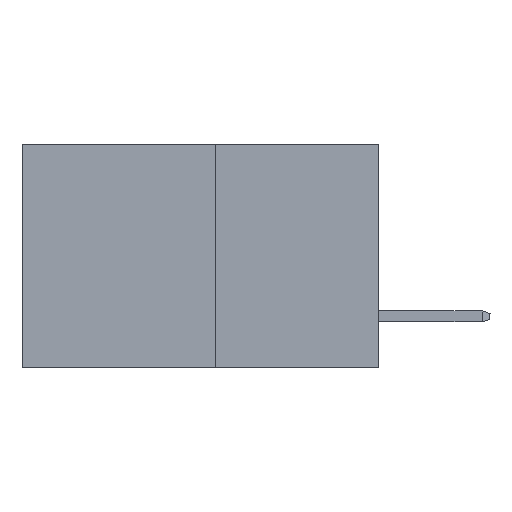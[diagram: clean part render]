
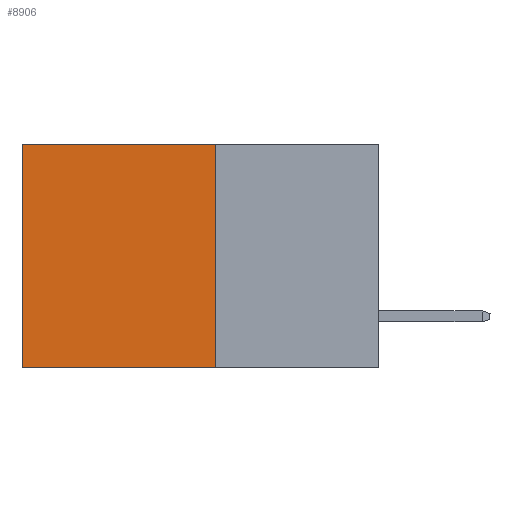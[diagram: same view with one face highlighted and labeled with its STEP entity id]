
A CAD part, left-side view. The second image highlights one B-rep face of the part: STEP entity #8906.
In plain terms, the highlighted planar face has unit normal (-1, 0, 0).
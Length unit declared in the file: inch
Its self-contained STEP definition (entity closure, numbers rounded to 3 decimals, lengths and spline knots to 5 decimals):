
#90 = ORIENTED_EDGE ( 'NONE', *, *, #6426, .F. ) ;
#382 = LINE ( 'NONE', #3004, #10397 ) ;
#418 = EDGE_CURVE ( 'NONE', #11303, #11766, #382, .T. ) ;
#494 = LINE ( 'NONE', #7568, #8043 ) ;
#1025 = LINE ( 'NONE', #3298, #10951 ) ;
#1126 = CARTESIAN_POINT ( 'NONE',  ( 0.277, 0.27, 0. ) ) ;
#1279 = EDGE_CURVE ( 'NONE', #1884, #5634, #1025, .T. ) ;
#1542 = ORIENTED_EDGE ( 'NONE', *, *, #1279, .T. ) ;
#1884 = VERTEX_POINT ( 'NONE', #11055 ) ;
#2034 = DIRECTION ( 'NONE',  ( 0., 1., 0. ) ) ;
#2112 = ORIENTED_EDGE ( 'NONE', *, *, #418, .F. ) ;
#2832 = CARTESIAN_POINT ( 'NONE',  ( 0.277, 0.59, -0.37 ) ) ;
#3004 = CARTESIAN_POINT ( 'NONE',  ( 0.277, 0.27, -0.37 ) ) ;
#3298 = CARTESIAN_POINT ( 'NONE',  ( 0.277, 0.59, -0.37 ) ) ;
#3558 = AXIS2_PLACEMENT_3D ( 'NONE', #8500, #8490, #8481 ) ;
#3573 = CARTESIAN_POINT ( 'NONE',  ( 0.277, 0.27, -0.37 ) ) ;
#4553 = FACE_OUTER_BOUND ( 'NONE', #7963, .T. ) ;
#4864 = EDGE_CURVE ( 'NONE', #11303, #1884, #494, .T. ) ;
#5371 = DIRECTION ( 'NONE',  ( 0., 0., -1. ) ) ;
#5634 = VERTEX_POINT ( 'NONE', #2832 ) ;
#5747 = DIRECTION ( 'NONE',  ( 0., 1., 0. ) ) ;
#6426 = EDGE_CURVE ( 'NONE', #11766, #5634, #8296, .T. ) ;
#7568 = CARTESIAN_POINT ( 'NONE',  ( 0.277, 0.27, 0. ) ) ;
#7963 = EDGE_LOOP ( 'NONE', ( #1542, #90, #2112, #10180 ) ) ;
#8020 = VECTOR ( 'NONE', #2034, 39.37008 ) ;
#8043 = VECTOR ( 'NONE', #5747, 39.37008 ) ;
#8296 = LINE ( 'NONE', #3573, #8020 ) ;
#8481 = DIRECTION ( 'NONE',  ( 0., 0., -1. ) ) ;
#8490 = DIRECTION ( 'NONE',  ( 1., 0., 0. ) ) ;
#8500 = CARTESIAN_POINT ( 'NONE',  ( 0.277, 0.27, -0.37 ) ) ;
#8552 = PLANE ( 'NONE',  #3558 ) ;
#8906 = ADVANCED_FACE ( 'NONE', ( #4553 ), #8552, .F. ) ;
#10180 = ORIENTED_EDGE ( 'NONE', *, *, #4864, .T. ) ;
#10215 = DIRECTION ( 'NONE',  ( 0., 0., -1. ) ) ;
#10397 = VECTOR ( 'NONE', #10215, 39.37008 ) ;
#10951 = VECTOR ( 'NONE', #5371, 39.37008 ) ;
#11055 = CARTESIAN_POINT ( 'NONE',  ( 0.277, 0.59, 0. ) ) ;
#11303 = VERTEX_POINT ( 'NONE', #1126 ) ;
#11766 = VERTEX_POINT ( 'NONE', #12363 ) ;
#12363 = CARTESIAN_POINT ( 'NONE',  ( 0.277, 0.27, -0.37 ) ) ;
